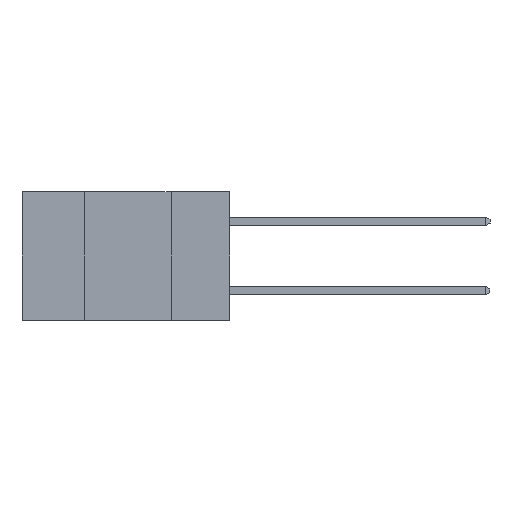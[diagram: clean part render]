
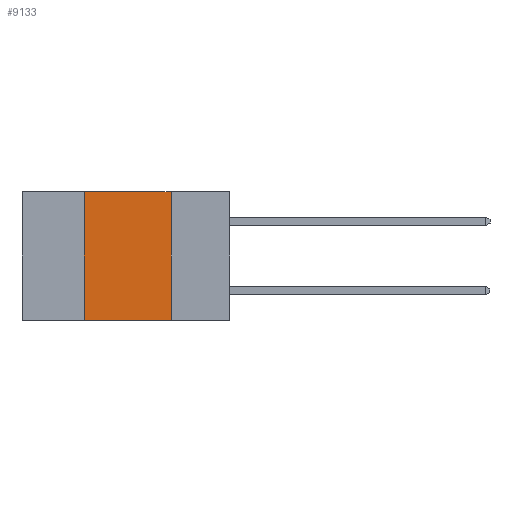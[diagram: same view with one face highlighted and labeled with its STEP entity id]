
A CAD part, left-side view. The second image highlights one B-rep face of the part: STEP entity #9133.
In plain terms, the highlighted planar face has unit normal (-1, 0, 0).
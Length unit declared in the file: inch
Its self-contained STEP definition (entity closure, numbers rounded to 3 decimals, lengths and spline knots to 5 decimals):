
#527 = DIRECTION ( 'NONE',  ( 0., -1., 0. ) ) ;
#858 = EDGE_CURVE ( 'NONE', #8188, #16440, #7287, .T. ) ;
#2004 = LINE ( 'NONE', #6971, #11385 ) ;
#2689 = DIRECTION ( 'NONE',  ( 0., 0., -1. ) ) ;
#4243 = VECTOR ( 'NONE', #8793, 39.37008 ) ;
#4265 = ORIENTED_EDGE ( 'NONE', *, *, #9231, .T. ) ;
#4342 = CARTESIAN_POINT ( 'NONE',  ( 0., 0.42, -0.37 ) ) ;
#4372 = DIRECTION ( 'NONE',  ( 1., 0., 0. ) ) ;
#5062 = LINE ( 'NONE', #7424, #4243 ) ;
#5335 = CARTESIAN_POINT ( 'NONE',  ( 0., 0.42, 0. ) ) ;
#6971 = CARTESIAN_POINT ( 'NONE',  ( 0., 0.6, 0. ) ) ;
#7287 = LINE ( 'NONE', #14269, #10846 ) ;
#7424 = CARTESIAN_POINT ( 'NONE',  ( 0., 0.42, 0. ) ) ;
#8188 = VERTEX_POINT ( 'NONE', #17014 ) ;
#8367 = EDGE_LOOP ( 'NONE', ( #16742, #8894, #14881, #4265 ) ) ;
#8793 = DIRECTION ( 'NONE',  ( 0., 0., 1. ) ) ;
#8894 = ORIENTED_EDGE ( 'NONE', *, *, #12841, .F. ) ;
#9133 = ADVANCED_FACE ( 'NONE', ( #16005 ), #9689, .F. ) ;
#9231 = EDGE_CURVE ( 'NONE', #12637, #16440, #14799, .T. ) ;
#9689 = PLANE ( 'NONE',  #12722 ) ;
#9853 = CARTESIAN_POINT ( 'NONE',  ( 0., 0.6, -0.37 ) ) ;
#10206 = CARTESIAN_POINT ( 'NONE',  ( 0., 0.17, -0.37 ) ) ;
#10846 = VECTOR ( 'NONE', #2689, 39.37008 ) ;
#11004 = DIRECTION ( 'NONE',  ( 0., -1., 0. ) ) ;
#11277 = VERTEX_POINT ( 'NONE', #5335 ) ;
#11385 = VECTOR ( 'NONE', #11004, 39.37008 ) ;
#12637 = VERTEX_POINT ( 'NONE', #4342 ) ;
#12722 = AXIS2_PLACEMENT_3D ( 'NONE', #13692, #4372, #13747 ) ;
#12841 = EDGE_CURVE ( 'NONE', #11277, #8188, #2004, .T. ) ;
#13692 = CARTESIAN_POINT ( 'NONE',  ( 0., 0.6, 0. ) ) ;
#13723 = EDGE_CURVE ( 'NONE', #12637, #11277, #5062, .T. ) ;
#13747 = DIRECTION ( 'NONE',  ( 0., 0., -1. ) ) ;
#14269 = CARTESIAN_POINT ( 'NONE',  ( 0., 0.17, 0. ) ) ;
#14799 = LINE ( 'NONE', #9853, #15213 ) ;
#14881 = ORIENTED_EDGE ( 'NONE', *, *, #13723, .F. ) ;
#15213 = VECTOR ( 'NONE', #527, 39.37008 ) ;
#16005 = FACE_OUTER_BOUND ( 'NONE', #8367, .T. ) ;
#16440 = VERTEX_POINT ( 'NONE', #10206 ) ;
#16742 = ORIENTED_EDGE ( 'NONE', *, *, #858, .F. ) ;
#17014 = CARTESIAN_POINT ( 'NONE',  ( 0., 0.17, 0. ) ) ;
